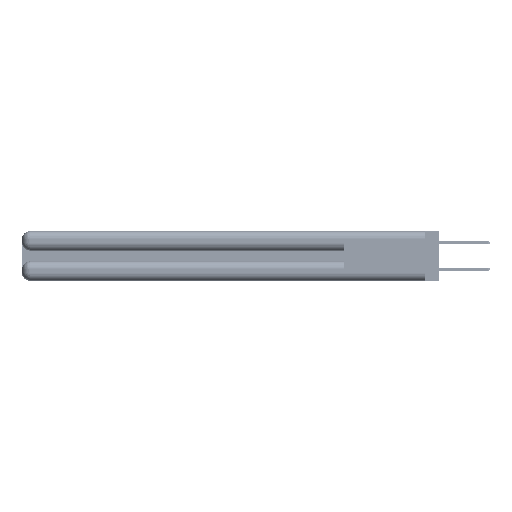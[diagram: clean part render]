
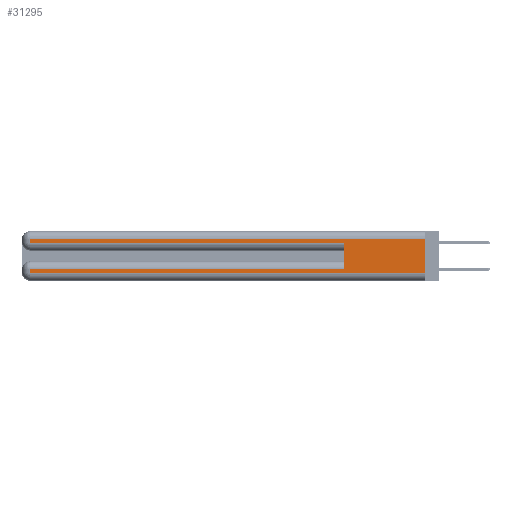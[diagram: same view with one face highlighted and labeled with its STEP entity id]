
A CAD part, left-side view. The second image highlights one B-rep face of the part: STEP entity #31295.
In plain terms, the highlighted planar face has unit normal (-1, 0, 0).
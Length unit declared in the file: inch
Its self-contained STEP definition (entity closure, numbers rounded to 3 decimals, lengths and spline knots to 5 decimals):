
#271 = LINE ( 'NONE', #5186, #2136 ) ;
#1844 = VECTOR ( 'NONE', #43019, 39.37008 ) ;
#1893 = EDGE_CURVE ( 'NONE', #9147, #9385, #271, .T. ) ;
#2136 = VECTOR ( 'NONE', #37690, 39.37008 ) ;
#2635 = VECTOR ( 'NONE', #42755, 39.37008 ) ;
#3249 = VECTOR ( 'NONE', #32579, 39.37008 ) ;
#3438 = DIRECTION ( 'NONE',  ( 0., 0., -1. ) ) ;
#4034 = ORIENTED_EDGE ( 'NONE', *, *, #11569, .F. ) ;
#5186 = CARTESIAN_POINT ( 'NONE',  ( 0., 2.94, 0.37 ) ) ;
#6357 = VECTOR ( 'NONE', #3438, 39.37008 ) ;
#7005 = CARTESIAN_POINT ( 'NONE',  ( 0., 0.6, 0.085 ) ) ;
#7655 = CARTESIAN_POINT ( 'NONE',  ( 0., 0., 0.37 ) ) ;
#9027 = EDGE_CURVE ( 'NONE', #9385, #26156, #35943, .T. ) ;
#9147 = VERTEX_POINT ( 'NONE', #29061 ) ;
#9385 = VERTEX_POINT ( 'NONE', #42207 ) ;
#9468 = VECTOR ( 'NONE', #38930, 39.37008 ) ;
#11028 = CARTESIAN_POINT ( 'NONE',  ( 0., 0., 0.37 ) ) ;
#11112 = CARTESIAN_POINT ( 'NONE',  ( 0., 0., 0.31 ) ) ;
#11269 = EDGE_CURVE ( 'NONE', #48275, #9147, #40140, .T. ) ;
#11569 = EDGE_CURVE ( 'NONE', #42241, #26156, #23210, .T. ) ;
#12125 = ORIENTED_EDGE ( 'NONE', *, *, #33473, .F. ) ;
#13315 = LINE ( 'NONE', #34683, #2635 ) ;
#13935 = LINE ( 'NONE', #40648, #3249 ) ;
#13974 = VECTOR ( 'NONE', #35935, 39.37008 ) ;
#14195 = FACE_OUTER_BOUND ( 'NONE', #49700, .T. ) ;
#15055 = DIRECTION ( 'NONE',  ( 1., 0., 0. ) ) ;
#16480 = EDGE_CURVE ( 'NONE', #22102, #51047, #13315, .T. ) ;
#16695 = EDGE_CURVE ( 'NONE', #51047, #29348, #13935, .T. ) ;
#18221 = EDGE_CURVE ( 'NONE', #42241, #22102, #49623, .T. ) ;
#18303 = LINE ( 'NONE', #7655, #6357 ) ;
#19056 = CARTESIAN_POINT ( 'NONE',  ( 0., 2.94, 0.085 ) ) ;
#19129 = CARTESIAN_POINT ( 'NONE',  ( 0., 0.6, 0.285 ) ) ;
#22102 = VERTEX_POINT ( 'NONE', #19056 ) ;
#23138 = DIRECTION ( 'NONE',  ( 0., 0., -1. ) ) ;
#23210 = LINE ( 'NONE', #39166, #1844 ) ;
#26156 = VERTEX_POINT ( 'NONE', #19129 ) ;
#28404 = AXIS2_PLACEMENT_3D ( 'NONE', #11028, #15055, #23138 ) ;
#29061 = CARTESIAN_POINT ( 'NONE',  ( 0., 2.94, 0.31 ) ) ;
#29348 = VERTEX_POINT ( 'NONE', #46328 ) ;
#31295 = ADVANCED_FACE ( 'NONE', ( #14195 ), #35415, .F. ) ;
#32083 = CARTESIAN_POINT ( 'NONE',  ( 0., 0., 0.285 ) ) ;
#32579 = DIRECTION ( 'NONE',  ( 0., -1., 0. ) ) ;
#33359 = ORIENTED_EDGE ( 'NONE', *, *, #16480, .T. ) ;
#33473 = EDGE_CURVE ( 'NONE', #48275, #29348, #18303, .T. ) ;
#33579 = DIRECTION ( 'NONE',  ( 0., 1., 0. ) ) ;
#34683 = CARTESIAN_POINT ( 'NONE',  ( 0., 2.94, 0.37 ) ) ;
#35415 = PLANE ( 'NONE',  #28404 ) ;
#35935 = DIRECTION ( 'NONE',  ( 0., -1., 0. ) ) ;
#35943 = LINE ( 'NONE', #32083, #13974 ) ;
#36647 = CARTESIAN_POINT ( 'NONE',  ( 0., 2.94, 0.06 ) ) ;
#37690 = DIRECTION ( 'NONE',  ( 0., 0., -1. ) ) ;
#38020 = ORIENTED_EDGE ( 'NONE', *, *, #1893, .T. ) ;
#38930 = DIRECTION ( 'NONE',  ( 0., 1., 0. ) ) ;
#39166 = CARTESIAN_POINT ( 'NONE',  ( 0., 0.6, 0.145 ) ) ;
#40140 = LINE ( 'NONE', #45124, #45733 ) ;
#40648 = CARTESIAN_POINT ( 'NONE',  ( 0., 0., 0.06 ) ) ;
#42207 = CARTESIAN_POINT ( 'NONE',  ( 0., 2.94, 0.285 ) ) ;
#42241 = VERTEX_POINT ( 'NONE', #7005 ) ;
#42755 = DIRECTION ( 'NONE',  ( 0., 0., -1. ) ) ;
#43019 = DIRECTION ( 'NONE',  ( 0., 0., 1. ) ) ;
#43372 = ORIENTED_EDGE ( 'NONE', *, *, #9027, .T. ) ;
#45124 = CARTESIAN_POINT ( 'NONE',  ( 0., 0., 0.31 ) ) ;
#45733 = VECTOR ( 'NONE', #33579, 39.37008 ) ;
#46328 = CARTESIAN_POINT ( 'NONE',  ( 0., 0., 0.06 ) ) ;
#46414 = CARTESIAN_POINT ( 'NONE',  ( 0., 0., 0.085 ) ) ;
#48275 = VERTEX_POINT ( 'NONE', #11112 ) ;
#49201 = ORIENTED_EDGE ( 'NONE', *, *, #16695, .T. ) ;
#49623 = LINE ( 'NONE', #46414, #9468 ) ;
#49700 = EDGE_LOOP ( 'NONE', ( #12125, #51280, #38020, #43372, #4034, #51869, #33359, #49201 ) ) ;
#51047 = VERTEX_POINT ( 'NONE', #36647 ) ;
#51280 = ORIENTED_EDGE ( 'NONE', *, *, #11269, .T. ) ;
#51869 = ORIENTED_EDGE ( 'NONE', *, *, #18221, .T. ) ;
